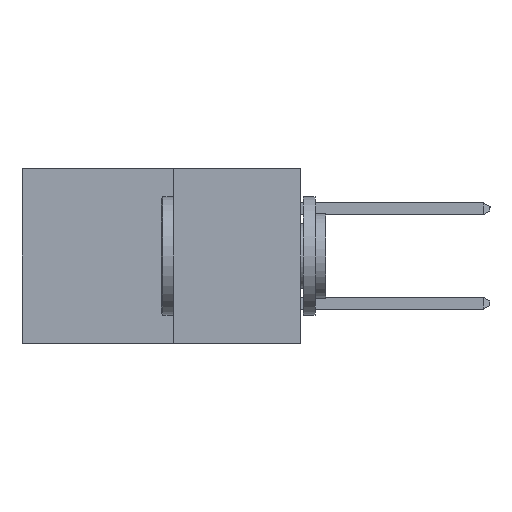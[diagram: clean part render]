
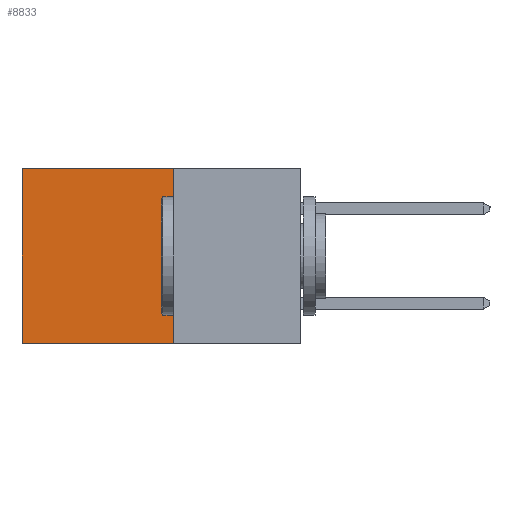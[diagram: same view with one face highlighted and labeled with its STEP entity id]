
A CAD part, left-side view. The second image highlights one B-rep face of the part: STEP entity #8833.
In plain terms, the highlighted planar face has unit normal (-1, 0, 0).
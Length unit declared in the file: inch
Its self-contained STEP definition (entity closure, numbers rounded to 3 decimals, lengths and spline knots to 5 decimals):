
#165 = ORIENTED_EDGE ( 'NONE', *, *, #10086, .T. ) ;
#623 = CARTESIAN_POINT ( 'NONE',  ( 0.277, 0.27, -0.37 ) ) ;
#1479 = FACE_OUTER_BOUND ( 'NONE', #1518, .T. ) ;
#1518 = EDGE_LOOP ( 'NONE', ( #165, #6363, #2368, #7459 ) ) ;
#1720 = EDGE_CURVE ( 'NONE', #8034, #7347, #9841, .T. ) ;
#2169 = CARTESIAN_POINT ( 'NONE',  ( 0.277, 0.27, 0. ) ) ;
#2368 = ORIENTED_EDGE ( 'NONE', *, *, #8271, .F. ) ;
#2624 = LINE ( 'NONE', #3801, #6778 ) ;
#3794 = DIRECTION ( 'NONE',  ( 0., 0., -1. ) ) ;
#3801 = CARTESIAN_POINT ( 'NONE',  ( 0.277, 0.27, -0.37 ) ) ;
#4056 = VECTOR ( 'NONE', #4993, 39.37008 ) ;
#4083 = VECTOR ( 'NONE', #4469, 39.37008 ) ;
#4461 = CARTESIAN_POINT ( 'NONE',  ( 0.277, 0.27, -0.37 ) ) ;
#4469 = DIRECTION ( 'NONE',  ( 0., 1., 0. ) ) ;
#4543 = CARTESIAN_POINT ( 'NONE',  ( 0.277, 0.59, -0.37 ) ) ;
#4888 = CARTESIAN_POINT ( 'NONE',  ( 0.277, 0.27, 0. ) ) ;
#4993 = DIRECTION ( 'NONE',  ( 0., 0., -1. ) ) ;
#5977 = VERTEX_POINT ( 'NONE', #623 ) ;
#6363 = ORIENTED_EDGE ( 'NONE', *, *, #8100, .F. ) ;
#6481 = DIRECTION ( 'NONE',  ( 0., 0., -1. ) ) ;
#6565 = DIRECTION ( 'NONE',  ( 1., 0., 0. ) ) ;
#6778 = VECTOR ( 'NONE', #3794, 39.37008 ) ;
#6829 = CARTESIAN_POINT ( 'NONE',  ( 0.277, 0.27, -0.37 ) ) ;
#6922 = PLANE ( 'NONE',  #8228 ) ;
#7347 = VERTEX_POINT ( 'NONE', #9117 ) ;
#7459 = ORIENTED_EDGE ( 'NONE', *, *, #1720, .T. ) ;
#7544 = VERTEX_POINT ( 'NONE', #8179 ) ;
#7915 = DIRECTION ( 'NONE',  ( 0., 1., 0. ) ) ;
#8034 = VERTEX_POINT ( 'NONE', #4888 ) ;
#8100 = EDGE_CURVE ( 'NONE', #5977, #7544, #9955, .T. ) ;
#8179 = CARTESIAN_POINT ( 'NONE',  ( 0.277, 0.59, -0.37 ) ) ;
#8220 = LINE ( 'NONE', #4543, #4056 ) ;
#8228 = AXIS2_PLACEMENT_3D ( 'NONE', #6829, #6565, #6481 ) ;
#8271 = EDGE_CURVE ( 'NONE', #8034, #5977, #2624, .T. ) ;
#8833 = ADVANCED_FACE ( 'NONE', ( #1479 ), #6922, .F. ) ;
#9117 = CARTESIAN_POINT ( 'NONE',  ( 0.277, 0.59, 0. ) ) ;
#9618 = VECTOR ( 'NONE', #7915, 39.37008 ) ;
#9841 = LINE ( 'NONE', #2169, #9618 ) ;
#9955 = LINE ( 'NONE', #4461, #4083 ) ;
#10086 = EDGE_CURVE ( 'NONE', #7347, #7544, #8220, .T. ) ;
